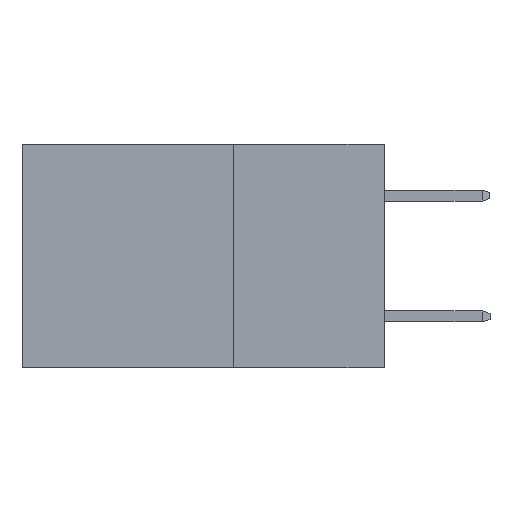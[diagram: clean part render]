
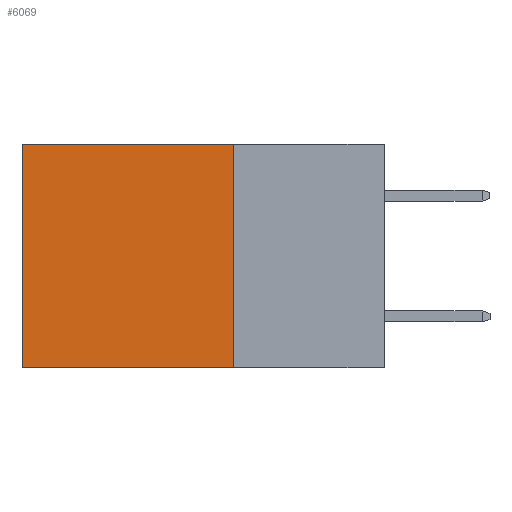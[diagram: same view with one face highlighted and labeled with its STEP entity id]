
A CAD part, left-side view. The second image highlights one B-rep face of the part: STEP entity #6069.
In plain terms, the highlighted planar face has unit normal (-1, 0, 0).
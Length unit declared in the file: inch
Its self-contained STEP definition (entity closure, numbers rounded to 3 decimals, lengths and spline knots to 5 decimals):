
#97 = EDGE_CURVE ( 'NONE', #3776, #2276, #6737, .T. ) ;
#190 = VECTOR ( 'NONE', #4743, 39.37008 ) ;
#396 = ORIENTED_EDGE ( 'NONE', *, *, #97, .T. ) ;
#417 = ORIENTED_EDGE ( 'NONE', *, *, #3097, .F. ) ;
#451 = CARTESIAN_POINT ( 'NONE',  ( 0.2615, 0.6, 0. ) ) ;
#525 = ORIENTED_EDGE ( 'NONE', *, *, #5827, .F. ) ;
#573 = ORIENTED_EDGE ( 'NONE', *, *, #6986, .T. ) ;
#614 = CARTESIAN_POINT ( 'NONE',  ( 0.2615, 0.25, -0.37 ) ) ;
#902 = CARTESIAN_POINT ( 'NONE',  ( 0.2615, 0.6, -0.37 ) ) ;
#1031 = DIRECTION ( 'NONE',  ( 0., 0., -1. ) ) ;
#1489 = DIRECTION ( 'NONE',  ( 0., 0., -1. ) ) ;
#1549 = CARTESIAN_POINT ( 'NONE',  ( 0.2615, 0.25, -0.37 ) ) ;
#2276 = VERTEX_POINT ( 'NONE', #4983 ) ;
#2556 = LINE ( 'NONE', #1549, #7539 ) ;
#2709 = LINE ( 'NONE', #4709, #190 ) ;
#3059 = VERTEX_POINT ( 'NONE', #4888 ) ;
#3097 = EDGE_CURVE ( 'NONE', #3720, #2276, #2709, .T. ) ;
#3720 = VERTEX_POINT ( 'NONE', #614 ) ;
#3776 = VERTEX_POINT ( 'NONE', #451 ) ;
#4121 = EDGE_LOOP ( 'NONE', ( #396, #417, #525, #573 ) ) ;
#4353 = AXIS2_PLACEMENT_3D ( 'NONE', #6311, #6301, #6268 ) ;
#4709 = CARTESIAN_POINT ( 'NONE',  ( 0.2615, 0.25, -0.37 ) ) ;
#4743 = DIRECTION ( 'NONE',  ( 0., 1., 0. ) ) ;
#4870 = VECTOR ( 'NONE', #6401, 39.37008 ) ;
#4888 = CARTESIAN_POINT ( 'NONE',  ( 0.2615, 0.25, 0. ) ) ;
#4983 = CARTESIAN_POINT ( 'NONE',  ( 0.2615, 0.6, -0.37 ) ) ;
#5034 = VECTOR ( 'NONE', #1031, 39.37008 ) ;
#5827 = EDGE_CURVE ( 'NONE', #3059, #3720, #2556, .T. ) ;
#6069 = ADVANCED_FACE ( 'NONE', ( #7548 ), #7204, .F. ) ;
#6268 = DIRECTION ( 'NONE',  ( 0., 0., -1. ) ) ;
#6301 = DIRECTION ( 'NONE',  ( 1., 0., 0. ) ) ;
#6311 = CARTESIAN_POINT ( 'NONE',  ( 0.2615, 0.25, -0.37 ) ) ;
#6401 = DIRECTION ( 'NONE',  ( 0., 1., 0. ) ) ;
#6452 = CARTESIAN_POINT ( 'NONE',  ( 0.2615, 0.25, 0. ) ) ;
#6561 = LINE ( 'NONE', #6452, #4870 ) ;
#6737 = LINE ( 'NONE', #902, #5034 ) ;
#6986 = EDGE_CURVE ( 'NONE', #3059, #3776, #6561, .T. ) ;
#7204 = PLANE ( 'NONE',  #4353 ) ;
#7539 = VECTOR ( 'NONE', #1489, 39.37008 ) ;
#7548 = FACE_OUTER_BOUND ( 'NONE', #4121, .T. ) ;
